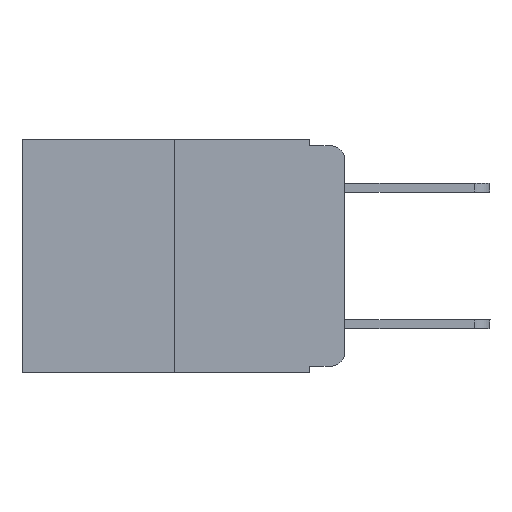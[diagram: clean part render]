
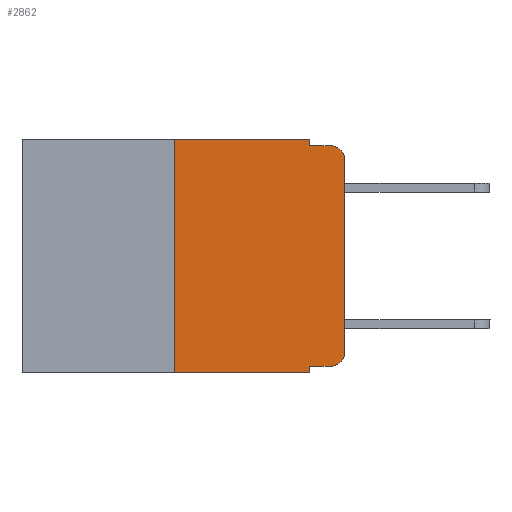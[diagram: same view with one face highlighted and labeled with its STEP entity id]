
A CAD part, left-side view. The second image highlights one B-rep face of the part: STEP entity #2862.
In plain terms, the highlighted planar face has unit normal (-1, 0, 0).
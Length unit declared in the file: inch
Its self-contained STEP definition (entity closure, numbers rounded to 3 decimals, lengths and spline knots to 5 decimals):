
#139 = VECTOR ( 'NONE', #7526, 39.37008 ) ;
#165 = CARTESIAN_POINT ( 'NONE',  ( 0., 0.051, -0.01 ) ) ;
#167 = EDGE_CURVE ( 'NONE', #9941, #6482, #8561, .T. ) ;
#194 = EDGE_CURVE ( 'NONE', #7891, #6482, #659, .T. ) ;
#527 = CARTESIAN_POINT ( 'NONE',  ( 0., 0.473, 0. ) ) ;
#538 = EDGE_CURVE ( 'NONE', #7889, #4799, #2239, .T. ) ;
#659 = CIRCLE ( 'NONE', #5481, 0.02 ) ;
#860 = CARTESIAN_POINT ( 'NONE',  ( 0., 0.02, -0.313 ) ) ;
#1021 = FACE_OUTER_BOUND ( 'NONE', #9036, .T. ) ;
#1173 = VECTOR ( 'NONE', #7381, 39.37008 ) ;
#1483 = EDGE_CURVE ( 'NONE', #6791, #4549, #3923, .T. ) ;
#1490 = DIRECTION ( 'NONE',  ( 1., 0., 0. ) ) ;
#1570 = ORIENTED_EDGE ( 'NONE', *, *, #194, .T. ) ;
#1689 = LINE ( 'NONE', #6937, #7466 ) ;
#1706 = CARTESIAN_POINT ( 'NONE',  ( 0., 0.25, 0. ) ) ;
#1990 = CARTESIAN_POINT ( 'NONE',  ( 0., 0.25, 0. ) ) ;
#2139 = LINE ( 'NONE', #3460, #139 ) ;
#2239 = LINE ( 'NONE', #527, #8685 ) ;
#2490 = VECTOR ( 'NONE', #3433, 39.37008 ) ;
#2776 = CARTESIAN_POINT ( 'NONE',  ( 0., 0.473, 0. ) ) ;
#2789 = CARTESIAN_POINT ( 'NONE',  ( 0., 0.051, -0.333 ) ) ;
#2850 = VERTEX_POINT ( 'NONE', #5420 ) ;
#2860 = CARTESIAN_POINT ( 'NONE',  ( 0., 0.02, -0.01 ) ) ;
#2862 = ADVANCED_FACE ( 'NONE', ( #1021 ), #7300, .F. ) ;
#3359 = CARTESIAN_POINT ( 'NONE',  ( 0., 0.02, -0.333 ) ) ;
#3367 = VERTEX_POINT ( 'NONE', #2789 ) ;
#3433 = DIRECTION ( 'NONE',  ( 0., 0., 1. ) ) ;
#3460 = CARTESIAN_POINT ( 'NONE',  ( 0., 0.051, -0.333 ) ) ;
#3567 = ORIENTED_EDGE ( 'NONE', *, *, #167, .F. ) ;
#3628 = LINE ( 'NONE', #9008, #10869 ) ;
#3725 = EDGE_CURVE ( 'NONE', #5448, #2850, #4649, .T. ) ;
#3784 = DIRECTION ( 'NONE',  ( 0., 0., 1. ) ) ;
#3923 = LINE ( 'NONE', #9879, #1173 ) ;
#4117 = DIRECTION ( 'NONE',  ( 0., -1., 0. ) ) ;
#4152 = CARTESIAN_POINT ( 'NONE',  ( 0., 0.02, -0.03 ) ) ;
#4442 = CARTESIAN_POINT ( 'NONE',  ( 0., 0., 0. ) ) ;
#4549 = VERTEX_POINT ( 'NONE', #7448 ) ;
#4649 = CIRCLE ( 'NONE', #8983, 0.02 ) ;
#4658 = ORIENTED_EDGE ( 'NONE', *, *, #10453, .F. ) ;
#4747 = VECTOR ( 'NONE', #4117, 39.37008 ) ;
#4760 = EDGE_CURVE ( 'NONE', #3367, #5448, #2139, .T. ) ;
#4799 = VERTEX_POINT ( 'NONE', #6734 ) ;
#4886 = DIRECTION ( 'NONE',  ( 0., 0., -1. ) ) ;
#4900 = DIRECTION ( 'NONE',  ( 0., -1., 0. ) ) ;
#5043 = DIRECTION ( 'NONE',  ( 0., 0., -1. ) ) ;
#5420 = CARTESIAN_POINT ( 'NONE',  ( 0., 0., -0.313 ) ) ;
#5448 = VERTEX_POINT ( 'NONE', #3359 ) ;
#5481 = AXIS2_PLACEMENT_3D ( 'NONE', #4152, #7451, #4886 ) ;
#5708 = DIRECTION ( 'NONE',  ( 0., 0., -1. ) ) ;
#5798 = EDGE_CURVE ( 'NONE', #2850, #7891, #8875, .T. ) ;
#5994 = AXIS2_PLACEMENT_3D ( 'NONE', #2776, #1490, #6943 ) ;
#6143 = CARTESIAN_POINT ( 'NONE',  ( 0., 0., -0.03 ) ) ;
#6482 = VERTEX_POINT ( 'NONE', #2860 ) ;
#6533 = CARTESIAN_POINT ( 'NONE',  ( 0., 0.25, -0.343 ) ) ;
#6615 = VECTOR ( 'NONE', #3784, 39.37008 ) ;
#6734 = CARTESIAN_POINT ( 'NONE',  ( 0., 0.051, 0. ) ) ;
#6791 = VERTEX_POINT ( 'NONE', #6533 ) ;
#6937 = CARTESIAN_POINT ( 'NONE',  ( 0., 0.051, 0. ) ) ;
#6943 = DIRECTION ( 'NONE',  ( 0., 0., -1. ) ) ;
#7215 = ORIENTED_EDGE ( 'NONE', *, *, #5798, .T. ) ;
#7300 = PLANE ( 'NONE',  #5994 ) ;
#7381 = DIRECTION ( 'NONE',  ( 0., -1., 0. ) ) ;
#7448 = CARTESIAN_POINT ( 'NONE',  ( 0., 0.051, -0.343 ) ) ;
#7451 = DIRECTION ( 'NONE',  ( -1., 0., 0. ) ) ;
#7466 = VECTOR ( 'NONE', #7791, 39.37008 ) ;
#7526 = DIRECTION ( 'NONE',  ( 0., -1., 0. ) ) ;
#7745 = ORIENTED_EDGE ( 'NONE', *, *, #538, .F. ) ;
#7791 = DIRECTION ( 'NONE',  ( 0., 0., -1. ) ) ;
#7889 = VERTEX_POINT ( 'NONE', #1990 ) ;
#7891 = VERTEX_POINT ( 'NONE', #6143 ) ;
#8012 = ORIENTED_EDGE ( 'NONE', *, *, #3725, .T. ) ;
#8534 = LINE ( 'NONE', #1706, #2490 ) ;
#8561 = LINE ( 'NONE', #10731, #4747 ) ;
#8685 = VECTOR ( 'NONE', #4900, 39.37008 ) ;
#8700 = ORIENTED_EDGE ( 'NONE', *, *, #8785, .F. ) ;
#8732 = EDGE_CURVE ( 'NONE', #6791, #7889, #8534, .T. ) ;
#8785 = EDGE_CURVE ( 'NONE', #3367, #4549, #1689, .T. ) ;
#8875 = LINE ( 'NONE', #4442, #6615 ) ;
#8983 = AXIS2_PLACEMENT_3D ( 'NONE', #860, #10909, #5043 ) ;
#9008 = CARTESIAN_POINT ( 'NONE',  ( 0., 0.051, 0. ) ) ;
#9036 = EDGE_LOOP ( 'NONE', ( #7215, #1570, #3567, #4658, #7745, #10736, #10627, #8700, #10796, #8012 ) ) ;
#9879 = CARTESIAN_POINT ( 'NONE',  ( 0., 0.473, -0.343 ) ) ;
#9941 = VERTEX_POINT ( 'NONE', #165 ) ;
#10453 = EDGE_CURVE ( 'NONE', #4799, #9941, #3628, .T. ) ;
#10627 = ORIENTED_EDGE ( 'NONE', *, *, #1483, .T. ) ;
#10731 = CARTESIAN_POINT ( 'NONE',  ( 0., 0.051, -0.01 ) ) ;
#10736 = ORIENTED_EDGE ( 'NONE', *, *, #8732, .F. ) ;
#10796 = ORIENTED_EDGE ( 'NONE', *, *, #4760, .T. ) ;
#10869 = VECTOR ( 'NONE', #5708, 39.37008 ) ;
#10909 = DIRECTION ( 'NONE',  ( -1., 0., 0. ) ) ;
